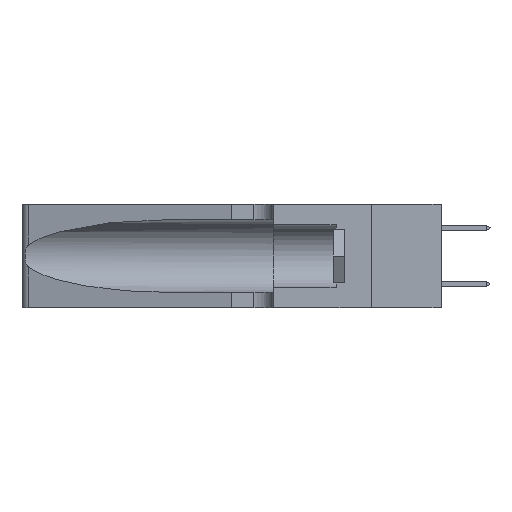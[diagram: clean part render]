
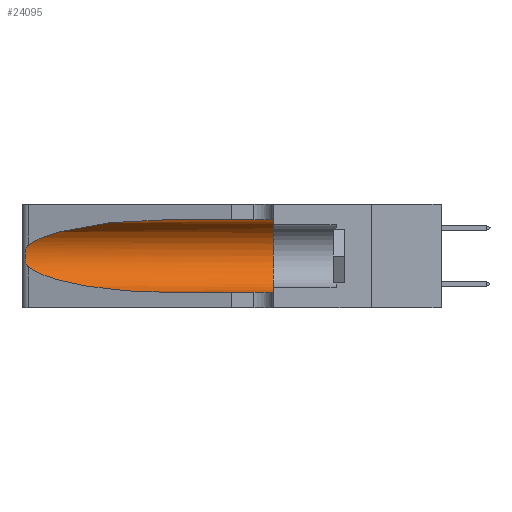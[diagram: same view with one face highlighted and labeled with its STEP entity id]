
A CAD part, left-side view. The second image highlights one B-rep face of the part: STEP entity #24095.
In plain terms, the highlighted cylindrical face has radius 3.308 mm (diameter 6.617 mm), a partial arc.
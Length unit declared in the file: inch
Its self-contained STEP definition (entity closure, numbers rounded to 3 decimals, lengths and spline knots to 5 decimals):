
#247 = DIRECTION ( 'NONE',  ( 0., -1., 0. ) ) ;
#324 = CARTESIAN_POINT ( 'NONE',  ( 0.25555, 1.22994, 0.2215 ) ) ;
#428 = CARTESIAN_POINT ( 'NONE',  ( 0.25555, 1.22993, 0.14849 ) ) ;
#820 = EDGE_CURVE ( 'NONE', #14820, #3244, #17909, .T. ) ;
#966 = AXIS2_PLACEMENT_3D ( 'NONE', #21875, #7319, #24308 ) ;
#2039 = AXIS2_PLACEMENT_3D ( 'NONE', #2316, #4741, #14512 ) ;
#2278 = VERTEX_POINT ( 'NONE', #22766 ) ;
#2316 = CARTESIAN_POINT ( 'NONE',  ( 0.1305, 1.61858, 0.185 ) ) ;
#3244 = VERTEX_POINT ( 'NONE', #30889 ) ;
#4337 = CARTESIAN_POINT ( 'NONE',  ( 0.18966, 0.96281, 0.31525 ) ) ;
#4741 = DIRECTION ( 'NONE',  ( 0., -1., 0. ) ) ;
#5150 = CARTESIAN_POINT ( 'NONE',  ( 0.25787, 1.23484, 0.2124 ) ) ;
#6812 = CARTESIAN_POINT ( 'NONE',  ( 0.25487, 1.22718, 0.22369 ) ) ;
#7232 = VECTOR ( 'NONE', #12030, 39.37008 ) ;
#7319 = DIRECTION ( 'NONE',  ( 0., 1., 0. ) ) ;
#7595 = VERTEX_POINT ( 'NONE', #17513 ) ;
#7644 = CARTESIAN_POINT ( 'NONE',  ( 0.26018, 1.23835, 0.19895 ) ) ;
#8861 = EDGE_CURVE ( 'NONE', #20380, #3244, #24118, .T. ) ;
#9527 = FACE_OUTER_BOUND ( 'NONE', #14348, .T. ) ;
#9619 = CARTESIAN_POINT ( 'NONE',  ( 0.1305, 0.35, 0.31525 ) ) ;
#9765 = ORIENTED_EDGE ( 'NONE', *, *, #17689, .T. ) ;
#10028 = CARTESIAN_POINT ( 'NONE',  ( 0.1305, 0.72297, 0.05475 ) ) ;
#10082 = EDGE_CURVE ( 'NONE', #7595, #20802, #13097, .T. ) ;
#10107 = CARTESIAN_POINT ( 'NONE',  ( 0.26075, 1.23896, 0.178 ) ) ;
#10254 = EDGE_CURVE ( 'NONE', #7595, #20380, #28408, .T. ) ;
#10321 = CARTESIAN_POINT ( 'NONE',  ( 0.1305, 0.72297, 0.05475 ) ) ;
#10692 =( BOUNDED_CURVE ( )  B_SPLINE_CURVE ( 3, ( #27121, #19960, #24826, #10321 ),
 .UNSPECIFIED., .F., .F. ) 
 B_SPLINE_CURVE_WITH_KNOTS ( ( 4, 4 ),
 ( 3.44316, 4.71239 ),
 .UNSPECIFIED. ) 
 CURVE ( )  GEOMETRIC_REPRESENTATION_ITEM ( )  RATIONAL_B_SPLINE_CURVE ( ( 1., 0.87, 0.87, 1. ) ) 
 REPRESENTATION_ITEM ( '' )  );
#11635 = ORIENTED_EDGE ( 'NONE', *, *, #820, .T. ) ;
#12030 = DIRECTION ( 'NONE',  ( 0., -1., 0. ) ) ;
#12224 = CARTESIAN_POINT ( 'NONE',  ( 0.1305, 1.61858, 0.31525 ) ) ;
#12621 = CARTESIAN_POINT ( 'NONE',  ( 0.25856, 1.23593, 0.16098 ) ) ;
#13097 =( BOUNDED_CURVE ( )  B_SPLINE_CURVE ( 3, ( #30944, #4337, #21383, #6812 ),
 .UNSPECIFIED., .F., .F. ) 
 B_SPLINE_CURVE_WITH_KNOTS ( ( 4, 4 ),
 ( 1.5708, 2.84003 ),
 .UNSPECIFIED. ) 
 CURVE ( )  GEOMETRIC_REPRESENTATION_ITEM ( )  RATIONAL_B_SPLINE_CURVE ( ( 1., 0.87, 0.87, 1. ) ) 
 REPRESENTATION_ITEM ( '' )  );
#13250 = ORIENTED_EDGE ( 'NONE', *, *, #17730, .T. ) ;
#13804 = CARTESIAN_POINT ( 'NONE',  ( 0.25487, 1.22718, 0.22369 ) ) ;
#14348 = EDGE_LOOP ( 'NONE', ( #15224, #9765, #13250, #11635, #18514, #21672 ) ) ;
#14512 = DIRECTION ( 'NONE',  ( 0., 0., -1. ) ) ;
#14820 = VERTEX_POINT ( 'NONE', #10028 ) ;
#15031 = CARTESIAN_POINT ( 'NONE',  ( 0.25639, 1.23186, 0.15144 ) ) ;
#15224 = ORIENTED_EDGE ( 'NONE', *, *, #10082, .T. ) ;
#15270 = CYLINDRICAL_SURFACE ( 'NONE', #2039, 0.13025 ) ;
#16347 = B_SPLINE_CURVE_WITH_KNOTS ( 'NONE', 3,
 ( #29231, #324, #19754, #5150, #22188, #7644, #24607, #10107, #27014, #12621, #29446, #15031, #428, #17440 ),
 .UNSPECIFIED., .F., .F.,
 ( 4, 2, 2, 2, 2, 2, 4 ),
 ( 0., 0.00027, 0.00053, 0.00107, 0.0016, 0.00187, 0.00214 ),
 .UNSPECIFIED. ) ;
#17440 = CARTESIAN_POINT ( 'NONE',  ( 0.25487, 1.22718, 0.14631 ) ) ;
#17513 = CARTESIAN_POINT ( 'NONE',  ( 0.1305, 0.72297, 0.31525 ) ) ;
#17689 = EDGE_CURVE ( 'NONE', #20802, #2278, #16347, .T. ) ;
#17730 = EDGE_CURVE ( 'NONE', #2278, #14820, #10692, .T. ) ;
#17909 = LINE ( 'NONE', #24150, #7232 ) ;
#18514 = ORIENTED_EDGE ( 'NONE', *, *, #8861, .F. ) ;
#19754 = CARTESIAN_POINT ( 'NONE',  ( 0.25639, 1.23184, 0.21858 ) ) ;
#19960 = CARTESIAN_POINT ( 'NONE',  ( 0.2373, 1.15595, 0.08982 ) ) ;
#20380 = VERTEX_POINT ( 'NONE', #9619 ) ;
#20802 = VERTEX_POINT ( 'NONE', #13804 ) ;
#21383 = CARTESIAN_POINT ( 'NONE',  ( 0.2373, 1.15595, 0.28018 ) ) ;
#21672 = ORIENTED_EDGE ( 'NONE', *, *, #10254, .F. ) ;
#21875 = CARTESIAN_POINT ( 'NONE',  ( 0.1305, 0.35, 0.185 ) ) ;
#22018 = VECTOR ( 'NONE', #247, 39.37008 ) ;
#22188 = CARTESIAN_POINT ( 'NONE',  ( 0.25854, 1.2359, 0.20912 ) ) ;
#22766 = CARTESIAN_POINT ( 'NONE',  ( 0.25487, 1.22718, 0.14631 ) ) ;
#24095 = ADVANCED_FACE ( 'NONE', ( #9527 ), #15270, .F. ) ;
#24118 = CIRCLE ( 'NONE', #966, 0.13025 ) ;
#24150 = CARTESIAN_POINT ( 'NONE',  ( 0.1305, 1.61858, 0.05475 ) ) ;
#24308 = DIRECTION ( 'NONE',  ( 0., 0., 1. ) ) ;
#24607 = CARTESIAN_POINT ( 'NONE',  ( 0.26075, 1.23896, 0.19203 ) ) ;
#24826 = CARTESIAN_POINT ( 'NONE',  ( 0.18966, 0.96281, 0.05475 ) ) ;
#27014 = CARTESIAN_POINT ( 'NONE',  ( 0.26017, 1.23833, 0.17102 ) ) ;
#27121 = CARTESIAN_POINT ( 'NONE',  ( 0.25487, 1.22718, 0.14631 ) ) ;
#28408 = LINE ( 'NONE', #12224, #22018 ) ;
#29231 = CARTESIAN_POINT ( 'NONE',  ( 0.25487, 1.22718, 0.22369 ) ) ;
#29446 = CARTESIAN_POINT ( 'NONE',  ( 0.25789, 1.23486, 0.15765 ) ) ;
#30889 = CARTESIAN_POINT ( 'NONE',  ( 0.1305, 0.35, 0.05475 ) ) ;
#30944 = CARTESIAN_POINT ( 'NONE',  ( 0.1305, 0.72297, 0.31525 ) ) ;
